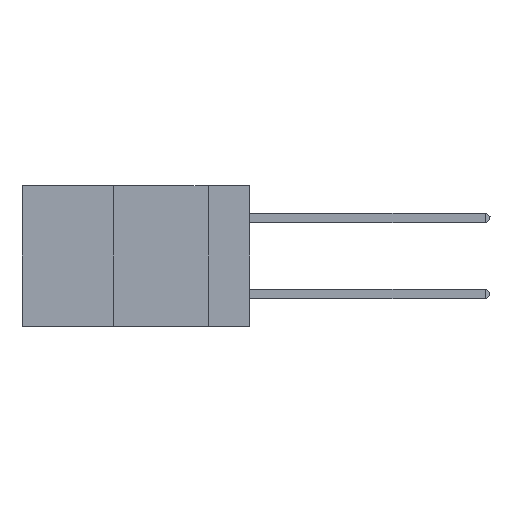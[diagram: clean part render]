
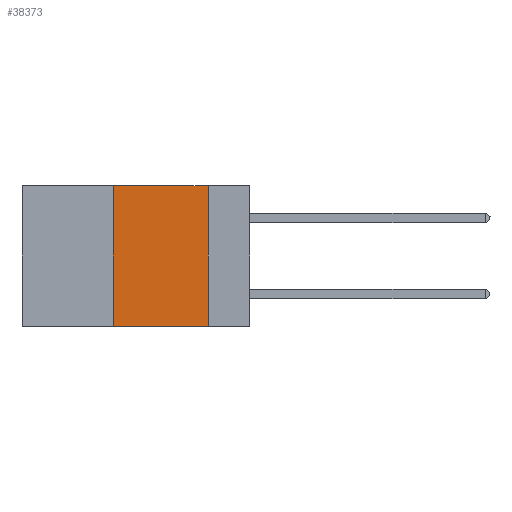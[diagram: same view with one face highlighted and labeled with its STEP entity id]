
A CAD part, left-side view. The second image highlights one B-rep face of the part: STEP entity #38373.
In plain terms, the highlighted planar face has unit normal (-1, 0, 0).
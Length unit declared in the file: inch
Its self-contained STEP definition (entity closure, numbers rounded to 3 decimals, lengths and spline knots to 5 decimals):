
#22 = DIRECTION ( 'NONE',  ( 0., 0., -1. ) ) ;
#277 = EDGE_CURVE ( 'NONE', #38785, #33286, #9772, .T. ) ;
#1880 = VECTOR ( 'NONE', #37303, 39.37008 ) ;
#2066 = CARTESIAN_POINT ( 'NONE',  ( 0., 0.11, 0. ) ) ;
#3052 = LINE ( 'NONE', #16224, #27350 ) ;
#6889 = EDGE_CURVE ( 'NONE', #38785, #31548, #7507, .T. ) ;
#6986 = EDGE_LOOP ( 'NONE', ( #28266, #27381, #9495, #38906 ) ) ;
#7507 = LINE ( 'NONE', #37522, #1880 ) ;
#9495 = ORIENTED_EDGE ( 'NONE', *, *, #6889, .F. ) ;
#9772 = LINE ( 'NONE', #22737, #19490 ) ;
#11772 = CARTESIAN_POINT ( 'NONE',  ( 0., 0.36, -0.37 ) ) ;
#13381 = EDGE_CURVE ( 'NONE', #26571, #33286, #3052, .T. ) ;
#14863 = PLANE ( 'NONE',  #18097 ) ;
#16224 = CARTESIAN_POINT ( 'NONE',  ( 0., 0.11, 0. ) ) ;
#16685 = DIRECTION ( 'NONE',  ( 0., -1., 0. ) ) ;
#18096 = DIRECTION ( 'NONE',  ( 0., 0., -1. ) ) ;
#18097 = AXIS2_PLACEMENT_3D ( 'NONE', #28239, #18525, #18096 ) ;
#18525 = DIRECTION ( 'NONE',  ( 1., 0., 0. ) ) ;
#19490 = VECTOR ( 'NONE', #22949, 39.37008 ) ;
#22737 = CARTESIAN_POINT ( 'NONE',  ( 0., 0.6, -0.37 ) ) ;
#22790 = CARTESIAN_POINT ( 'NONE',  ( 0., 0.36, 0. ) ) ;
#22949 = DIRECTION ( 'NONE',  ( 0., -1., 0. ) ) ;
#23854 = CARTESIAN_POINT ( 'NONE',  ( 0., 0.11, -0.37 ) ) ;
#24357 = FACE_OUTER_BOUND ( 'NONE', #6986, .T. ) ;
#26571 = VERTEX_POINT ( 'NONE', #2066 ) ;
#26589 = CARTESIAN_POINT ( 'NONE',  ( 0., 0.6, 0. ) ) ;
#27350 = VECTOR ( 'NONE', #22, 39.37008 ) ;
#27381 = ORIENTED_EDGE ( 'NONE', *, *, #28928, .F. ) ;
#28239 = CARTESIAN_POINT ( 'NONE',  ( 0., 0.6, 0. ) ) ;
#28266 = ORIENTED_EDGE ( 'NONE', *, *, #13381, .F. ) ;
#28928 = EDGE_CURVE ( 'NONE', #31548, #26571, #33508, .T. ) ;
#31548 = VERTEX_POINT ( 'NONE', #22790 ) ;
#33286 = VERTEX_POINT ( 'NONE', #23854 ) ;
#33508 = LINE ( 'NONE', #26589, #35423 ) ;
#35423 = VECTOR ( 'NONE', #16685, 39.37008 ) ;
#37303 = DIRECTION ( 'NONE',  ( 0., 0., 1. ) ) ;
#37522 = CARTESIAN_POINT ( 'NONE',  ( 0., 0.36, 0. ) ) ;
#38373 = ADVANCED_FACE ( 'NONE', ( #24357 ), #14863, .F. ) ;
#38785 = VERTEX_POINT ( 'NONE', #11772 ) ;
#38906 = ORIENTED_EDGE ( 'NONE', *, *, #277, .T. ) ;
